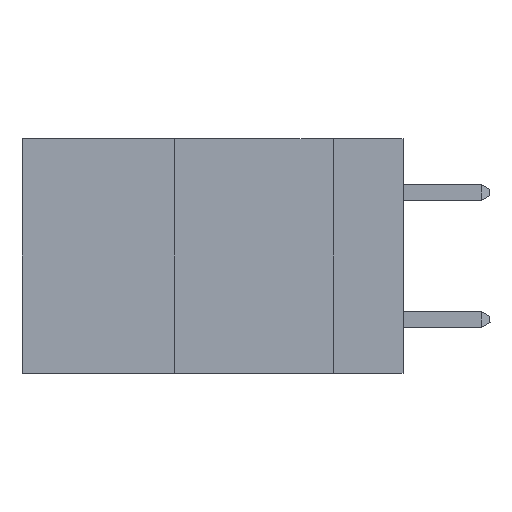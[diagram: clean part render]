
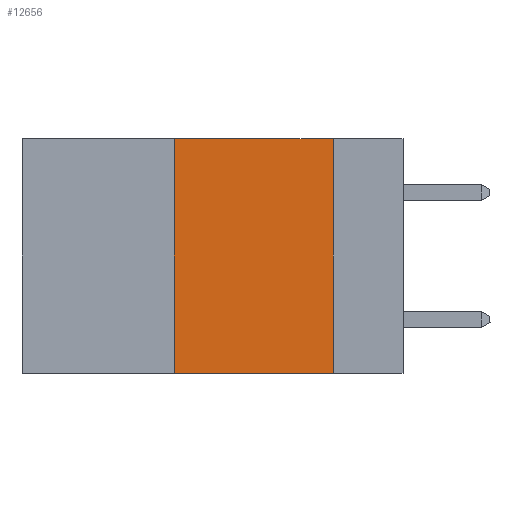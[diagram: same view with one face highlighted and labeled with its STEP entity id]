
A CAD part, left-side view. The second image highlights one B-rep face of the part: STEP entity #12656.
In plain terms, the highlighted planar face has unit normal (-1, 0, 0).
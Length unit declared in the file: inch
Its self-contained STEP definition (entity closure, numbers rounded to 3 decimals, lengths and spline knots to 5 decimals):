
#1510 = DIRECTION ( 'NONE',  ( 0., 0., -1. ) ) ;
#2757 = DIRECTION ( 'NONE',  ( 1., 0., 0. ) ) ;
#3562 = VERTEX_POINT ( 'NONE', #17896 ) ;
#4189 = DIRECTION ( 'NONE',  ( 0., 0., 1. ) ) ;
#5356 = CARTESIAN_POINT ( 'NONE',  ( 0., 0.6, 0. ) ) ;
#5807 = LINE ( 'NONE', #17313, #19603 ) ;
#7073 = DIRECTION ( 'NONE',  ( 0., -1., 0. ) ) ;
#7123 = CARTESIAN_POINT ( 'NONE',  ( 0., 0.6, -0.37 ) ) ;
#7166 = LINE ( 'NONE', #5356, #12846 ) ;
#7270 = ORIENTED_EDGE ( 'NONE', *, *, #9790, .F. ) ;
#7381 = VERTEX_POINT ( 'NONE', #22617 ) ;
#7643 = EDGE_CURVE ( 'NONE', #7381, #3562, #19130, .T. ) ;
#8110 = CARTESIAN_POINT ( 'NONE',  ( 0., 0.6, 0. ) ) ;
#8269 = PLANE ( 'NONE',  #18450 ) ;
#9790 = EDGE_CURVE ( 'NONE', #7381, #14269, #19075, .T. ) ;
#10096 = EDGE_CURVE ( 'NONE', #14269, #19474, #7166, .T. ) ;
#12560 = CARTESIAN_POINT ( 'NONE',  ( 0., 0.36, 0. ) ) ;
#12656 = ADVANCED_FACE ( 'NONE', ( #19097 ), #8269, .F. ) ;
#12846 = VECTOR ( 'NONE', #7073, 39.37008 ) ;
#13809 = VECTOR ( 'NONE', #16199, 39.37008 ) ;
#14269 = VERTEX_POINT ( 'NONE', #23250 ) ;
#14859 = EDGE_LOOP ( 'NONE', ( #18661, #17494, #7270, #16581 ) ) ;
#16199 = DIRECTION ( 'NONE',  ( 0., -1., 0. ) ) ;
#16581 = ORIENTED_EDGE ( 'NONE', *, *, #7643, .T. ) ;
#17313 = CARTESIAN_POINT ( 'NONE',  ( 0., 0.11, 0. ) ) ;
#17494 = ORIENTED_EDGE ( 'NONE', *, *, #10096, .F. ) ;
#17896 = CARTESIAN_POINT ( 'NONE',  ( 0., 0.11, -0.37 ) ) ;
#18450 = AXIS2_PLACEMENT_3D ( 'NONE', #8110, #2757, #18972 ) ;
#18509 = VECTOR ( 'NONE', #4189, 39.37008 ) ;
#18661 = ORIENTED_EDGE ( 'NONE', *, *, #19205, .F. ) ;
#18972 = DIRECTION ( 'NONE',  ( 0., 0., -1. ) ) ;
#19075 = LINE ( 'NONE', #12560, #18509 ) ;
#19097 = FACE_OUTER_BOUND ( 'NONE', #14859, .T. ) ;
#19130 = LINE ( 'NONE', #7123, #13809 ) ;
#19205 = EDGE_CURVE ( 'NONE', #19474, #3562, #5807, .T. ) ;
#19474 = VERTEX_POINT ( 'NONE', #20683 ) ;
#19603 = VECTOR ( 'NONE', #1510, 39.37008 ) ;
#20683 = CARTESIAN_POINT ( 'NONE',  ( 0., 0.11, 0. ) ) ;
#22617 = CARTESIAN_POINT ( 'NONE',  ( 0., 0.36, -0.37 ) ) ;
#23250 = CARTESIAN_POINT ( 'NONE',  ( 0., 0.36, 0. ) ) ;
